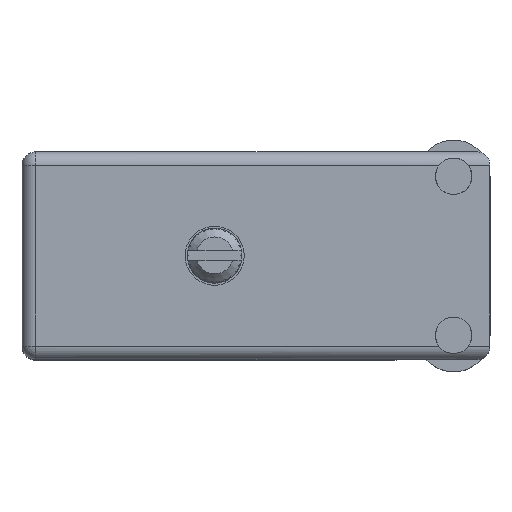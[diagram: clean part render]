
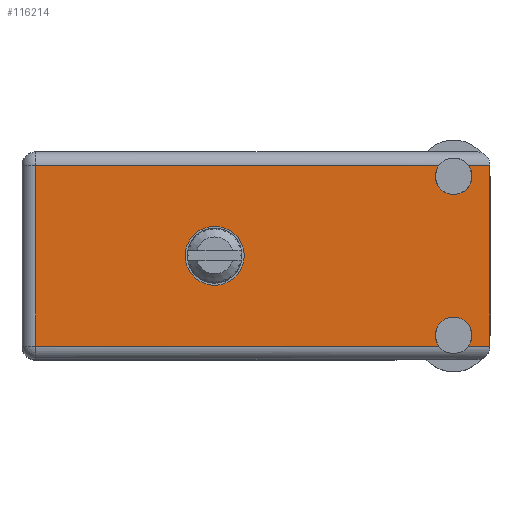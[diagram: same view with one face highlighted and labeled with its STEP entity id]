
A CAD part, top view. The second image highlights one B-rep face of the part: STEP entity #116214.
In plain terms, the highlighted face is planar.
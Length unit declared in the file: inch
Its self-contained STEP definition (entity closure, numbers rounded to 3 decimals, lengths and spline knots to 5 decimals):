
#1939 = VECTOR ( 'NONE', #175748, 39.37008 ) ;
#2016 = EDGE_CURVE ( 'NONE', #176195, #108802, #78786, .T. ) ;
#2114 = ORIENTED_EDGE ( 'NONE', *, *, #117720, .T. ) ;
#2629 = EDGE_LOOP ( 'NONE', ( #2114, #51639, #15596, #143595, #161530, #78633, #56809, #194865, #54392, #11703 ) ) ;
#6212 = CARTESIAN_POINT ( 'NONE',  ( 0.6625, 0.906, -0.3575 ) ) ;
#6756 = LINE ( 'NONE', #21494, #72809 ) ;
#7577 = DIRECTION ( 'NONE',  ( 0., 1., 0. ) ) ;
#11703 = ORIENTED_EDGE ( 'NONE', *, *, #193573, .T. ) ;
#13501 = EDGE_CURVE ( 'NONE', #108802, #176195, #19170, .T. ) ;
#14005 = DIRECTION ( 'NONE',  ( 0., 0., 1. ) ) ;
#14312 = AXIS2_PLACEMENT_3D ( 'NONE', #87333, #191989, #175507 ) ;
#14419 = CARTESIAN_POINT ( 'NONE',  ( 1.484, 0.906, -0.084 ) ) ;
#15596 = ORIENTED_EDGE ( 'NONE', *, *, #118156, .F. ) ;
#16367 = LINE ( 'NONE', #154578, #127202 ) ;
#18657 = VERTEX_POINT ( 'NONE', #193671 ) ;
#19170 = CIRCLE ( 'NONE', #135389, 0.1015 ) ;
#20841 = AXIS2_PLACEMENT_3D ( 'NONE', #108952, #124138, #48976 ) ;
#21494 = CARTESIAN_POINT ( 'NONE',  ( 1.609, 0.906, -0.047 ) ) ;
#23717 = EDGE_CURVE ( 'NONE', #131252, #123088, #67491, .T. ) ;
#26104 = AXIS2_PLACEMENT_3D ( 'NONE', #53005, #7577, #143243 ) ;
#28521 = VECTOR ( 'NONE', #141477, 39.37008 ) ;
#30714 = CARTESIAN_POINT ( 'NONE',  ( 0.6625, 0.906, -0.256 ) ) ;
#31821 = CARTESIAN_POINT ( 'NONE',  ( 0.6625, 0.906, -0.459 ) ) ;
#37774 = CARTESIAN_POINT ( 'NONE',  ( 1.53437, 0.906, -0.047 ) ) ;
#38081 = CARTESIAN_POINT ( 'NONE',  ( 1.484, 0.906, -0.1465 ) ) ;
#38243 = DIRECTION ( 'NONE',  ( 0., 1., 0. ) ) ;
#45310 = VERTEX_POINT ( 'NONE', #190635 ) ;
#48581 = DIRECTION ( 'NONE',  ( -1., 0., 0. ) ) ;
#48976 = DIRECTION ( 'NONE',  ( 0., 0., 1. ) ) ;
#51603 = DIRECTION ( 'NONE',  ( 0., 1., 0. ) ) ;
#51639 = ORIENTED_EDGE ( 'NONE', *, *, #114833, .F. ) ;
#53005 = CARTESIAN_POINT ( 'NONE',  ( 1.484, 0.906, -0.631 ) ) ;
#54392 = ORIENTED_EDGE ( 'NONE', *, *, #128087, .T. ) ;
#56694 = VERTEX_POINT ( 'NONE', #38081 ) ;
#56809 = ORIENTED_EDGE ( 'NONE', *, *, #157100, .F. ) ;
#59445 = EDGE_LOOP ( 'NONE', ( #172105, #104411 ) ) ;
#59860 = AXIS2_PLACEMENT_3D ( 'NONE', #14419, #151388, #61183 ) ;
#61183 = DIRECTION ( 'NONE',  ( 0., 0., 1. ) ) ;
#63527 = PLANE ( 'NONE',  #20841 ) ;
#67491 = CIRCLE ( 'NONE', #14312, 0.0625 ) ;
#70230 = LINE ( 'NONE', #162544, #1939 ) ;
#70884 = AXIS2_PLACEMENT_3D ( 'NONE', #194481, #104314, #14005 ) ;
#71132 = LINE ( 'NONE', #111180, #28521 ) ;
#71325 = CARTESIAN_POINT ( 'NONE',  ( 1.43363, 0.906, -0.047 ) ) ;
#72809 = VECTOR ( 'NONE', #189413, 39.37008 ) ;
#75754 = EDGE_CURVE ( 'NONE', #98570, #149499, #70230, .T. ) ;
#78633 = ORIENTED_EDGE ( 'NONE', *, *, #84933, .T. ) ;
#78786 = CIRCLE ( 'NONE', #80026, 0.1015 ) ;
#80026 = AXIS2_PLACEMENT_3D ( 'NONE', #96224, #38243, #96882 ) ;
#84933 = EDGE_CURVE ( 'NONE', #98570, #18657, #16367, .T. ) ;
#86003 = DIRECTION ( 'NONE',  ( 0., 0., 1. ) ) ;
#87333 = CARTESIAN_POINT ( 'NONE',  ( 1.484, 0.906, -0.631 ) ) ;
#89252 = CIRCLE ( 'NONE', #70884, 0.0625 ) ;
#96224 = CARTESIAN_POINT ( 'NONE',  ( 0.6625, 0.906, -0.3575 ) ) ;
#96882 = DIRECTION ( 'NONE',  ( 0., 0., 1. ) ) ;
#98570 = VERTEX_POINT ( 'NONE', #158030 ) ;
#104314 = DIRECTION ( 'NONE',  ( 0., 1., 0. ) ) ;
#104411 = ORIENTED_EDGE ( 'NONE', *, *, #2016, .F. ) ;
#104419 = FACE_OUTER_BOUND ( 'NONE', #2629, .T. ) ;
#108802 = VERTEX_POINT ( 'NONE', #30714 ) ;
#108952 = CARTESIAN_POINT ( 'NONE',  ( 0., 0.906, -0.715 ) ) ;
#109451 = CIRCLE ( 'NONE', #26104, 0.0625 ) ;
#111180 = CARTESIAN_POINT ( 'NONE',  ( 0.047, 0.906, -0.715 ) ) ;
#114532 = CARTESIAN_POINT ( 'NONE',  ( 1.609, 0.906, -0.047 ) ) ;
#114833 = EDGE_CURVE ( 'NONE', #56694, #170438, #189378, .T. ) ;
#116214 = ADVANCED_FACE ( 'NONE', ( #123282, #104419 ), #63527, .T. ) ;
#117720 = EDGE_CURVE ( 'NONE', #45310, #170438, #6756, .T. ) ;
#118156 = EDGE_CURVE ( 'NONE', #150261, #56694, #89252, .T. ) ;
#119570 = VERTEX_POINT ( 'NONE', #137882 ) ;
#123088 = VERTEX_POINT ( 'NONE', #126210 ) ;
#123282 = FACE_BOUND ( 'NONE', #59445, .T. ) ;
#123444 = LINE ( 'NONE', #140120, #151546 ) ;
#124138 = DIRECTION ( 'NONE',  ( 0., 1., 0. ) ) ;
#126210 = CARTESIAN_POINT ( 'NONE',  ( 1.484, 0.906, -0.5685 ) ) ;
#127202 = VECTOR ( 'NONE', #48581, 39.37008 ) ;
#128087 = EDGE_CURVE ( 'NONE', #131252, #119570, #160804, .T. ) ;
#131252 = VERTEX_POINT ( 'NONE', #178618 ) ;
#135389 = AXIS2_PLACEMENT_3D ( 'NONE', #6212, #51603, #86003 ) ;
#137882 = CARTESIAN_POINT ( 'NONE',  ( 0.047, 0.906, -0.668 ) ) ;
#140120 = CARTESIAN_POINT ( 'NONE',  ( 1.609, 0.906, -0.047 ) ) ;
#141477 = DIRECTION ( 'NONE',  ( 0., 0., 1. ) ) ;
#143243 = DIRECTION ( 'NONE',  ( 0., 0., 1. ) ) ;
#143595 = ORIENTED_EDGE ( 'NONE', *, *, #158072, .T. ) ;
#149499 = VERTEX_POINT ( 'NONE', #114532 ) ;
#150261 = VERTEX_POINT ( 'NONE', #37774 ) ;
#151388 = DIRECTION ( 'NONE',  ( 0., 1., 0. ) ) ;
#151546 = VECTOR ( 'NONE', #155193, 39.37008 ) ;
#154578 = CARTESIAN_POINT ( 'NONE',  ( 0., 0.906, -0.668 ) ) ;
#155193 = DIRECTION ( 'NONE',  ( 1., 0., 0. ) ) ;
#157100 = EDGE_CURVE ( 'NONE', #123088, #18657, #109451, .T. ) ;
#157793 = DIRECTION ( 'NONE',  ( -1., 0., 0. ) ) ;
#158030 = CARTESIAN_POINT ( 'NONE',  ( 1.609, 0.906, -0.668 ) ) ;
#158072 = EDGE_CURVE ( 'NONE', #150261, #149499, #123444, .T. ) ;
#160804 = LINE ( 'NONE', #188103, #174997 ) ;
#161530 = ORIENTED_EDGE ( 'NONE', *, *, #75754, .F. ) ;
#162544 = CARTESIAN_POINT ( 'NONE',  ( 1.609, 0.906, 0. ) ) ;
#170438 = VERTEX_POINT ( 'NONE', #71325 ) ;
#172105 = ORIENTED_EDGE ( 'NONE', *, *, #13501, .F. ) ;
#174997 = VECTOR ( 'NONE', #157793, 39.37008 ) ;
#175507 = DIRECTION ( 'NONE',  ( 0., 0., 1. ) ) ;
#175748 = DIRECTION ( 'NONE',  ( 0., 0., 1. ) ) ;
#176195 = VERTEX_POINT ( 'NONE', #31821 ) ;
#178618 = CARTESIAN_POINT ( 'NONE',  ( 1.43363, 0.906, -0.668 ) ) ;
#188103 = CARTESIAN_POINT ( 'NONE',  ( 0., 0.906, -0.668 ) ) ;
#189378 = CIRCLE ( 'NONE', #59860, 0.0625 ) ;
#189413 = DIRECTION ( 'NONE',  ( 1., 0., 0. ) ) ;
#190635 = CARTESIAN_POINT ( 'NONE',  ( 0.047, 0.906, -0.047 ) ) ;
#191989 = DIRECTION ( 'NONE',  ( 0., 1., 0. ) ) ;
#193573 = EDGE_CURVE ( 'NONE', #119570, #45310, #71132, .T. ) ;
#193671 = CARTESIAN_POINT ( 'NONE',  ( 1.53437, 0.906, -0.668 ) ) ;
#194481 = CARTESIAN_POINT ( 'NONE',  ( 1.484, 0.906, -0.084 ) ) ;
#194865 = ORIENTED_EDGE ( 'NONE', *, *, #23717, .F. ) ;
